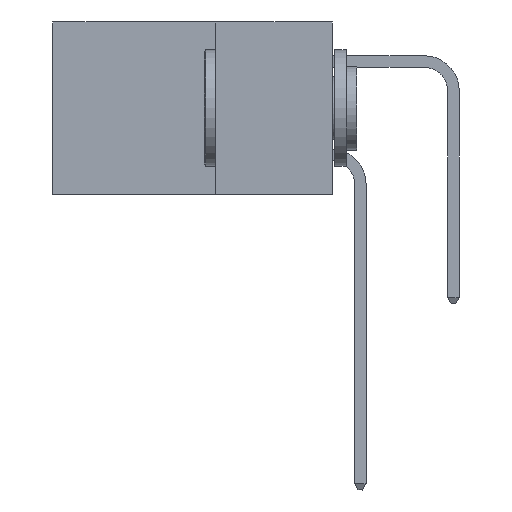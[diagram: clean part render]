
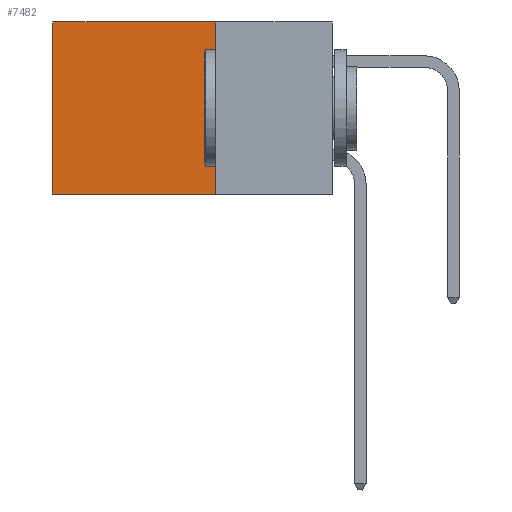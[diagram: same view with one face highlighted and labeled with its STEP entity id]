
A CAD part, left-side view. The second image highlights one B-rep face of the part: STEP entity #7482.
In plain terms, the highlighted planar face has unit normal (-1, 0, 0).
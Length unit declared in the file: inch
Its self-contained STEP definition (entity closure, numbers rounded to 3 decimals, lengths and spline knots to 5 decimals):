
#745 = LINE ( 'NONE', #20407, #16163 ) ;
#1184 = FACE_OUTER_BOUND ( 'NONE', #19672, .T. ) ;
#1680 = DIRECTION ( 'NONE',  ( 0., 0., -1. ) ) ;
#2969 = EDGE_CURVE ( 'NONE', #7125, #7550, #745, .T. ) ;
#3518 = ORIENTED_EDGE ( 'NONE', *, *, #8425, .T. ) ;
#4613 = VECTOR ( 'NONE', #1680, 39.37008 ) ;
#4695 = LINE ( 'NONE', #23527, #14702 ) ;
#5000 = DIRECTION ( 'NONE',  ( 1., 0., 0. ) ) ;
#5618 = VERTEX_POINT ( 'NONE', #19025 ) ;
#6021 = VERTEX_POINT ( 'NONE', #10254 ) ;
#6405 = ORIENTED_EDGE ( 'NONE', *, *, #22158, .F. ) ;
#6453 = EDGE_CURVE ( 'NONE', #6021, #5618, #4695, .T. ) ;
#7125 = VERTEX_POINT ( 'NONE', #15415 ) ;
#7482 = ADVANCED_FACE ( 'NONE', ( #1184 ), #14960, .F. ) ;
#7550 = VERTEX_POINT ( 'NONE', #9214 ) ;
#8425 = EDGE_CURVE ( 'NONE', #5618, #7550, #15241, .T. ) ;
#9214 = CARTESIAN_POINT ( 'NONE',  ( 0.298, 0.6, -0.37 ) ) ;
#10254 = CARTESIAN_POINT ( 'NONE',  ( 0.298, 0.25, 0. ) ) ;
#11222 = AXIS2_PLACEMENT_3D ( 'NONE', #16989, #5000, #19027 ) ;
#11735 = CARTESIAN_POINT ( 'NONE',  ( 0.298, 0.25, 0. ) ) ;
#12080 = DIRECTION ( 'NONE',  ( 0., 1., 0. ) ) ;
#14702 = VECTOR ( 'NONE', #19616, 39.37008 ) ;
#14960 = PLANE ( 'NONE',  #11222 ) ;
#15241 = LINE ( 'NONE', #25687, #4613 ) ;
#15415 = CARTESIAN_POINT ( 'NONE',  ( 0.298, 0.25, -0.37 ) ) ;
#16163 = VECTOR ( 'NONE', #12080, 39.37008 ) ;
#16989 = CARTESIAN_POINT ( 'NONE',  ( 0.298, 0.25, 0. ) ) ;
#19025 = CARTESIAN_POINT ( 'NONE',  ( 0.298, 0.6, 0. ) ) ;
#19027 = DIRECTION ( 'NONE',  ( 0., 0., -1. ) ) ;
#19616 = DIRECTION ( 'NONE',  ( 0., 1., 0. ) ) ;
#19672 = EDGE_LOOP ( 'NONE', ( #3518, #25141, #6405, #24035 ) ) ;
#20407 = CARTESIAN_POINT ( 'NONE',  ( 0.298, 0.25, -0.37 ) ) ;
#20635 = LINE ( 'NONE', #11735, #24673 ) ;
#21722 = DIRECTION ( 'NONE',  ( 0., 0., -1. ) ) ;
#22158 = EDGE_CURVE ( 'NONE', #6021, #7125, #20635, .T. ) ;
#23527 = CARTESIAN_POINT ( 'NONE',  ( 0.298, 0.25, 0. ) ) ;
#24035 = ORIENTED_EDGE ( 'NONE', *, *, #6453, .T. ) ;
#24673 = VECTOR ( 'NONE', #21722, 39.37008 ) ;
#25141 = ORIENTED_EDGE ( 'NONE', *, *, #2969, .F. ) ;
#25687 = CARTESIAN_POINT ( 'NONE',  ( 0.298, 0.6, 0. ) ) ;
